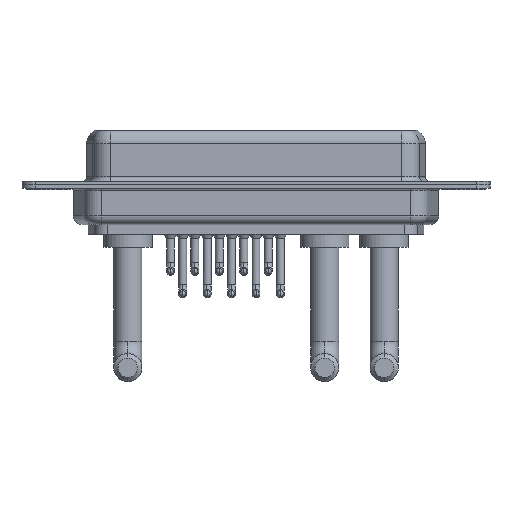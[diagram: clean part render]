
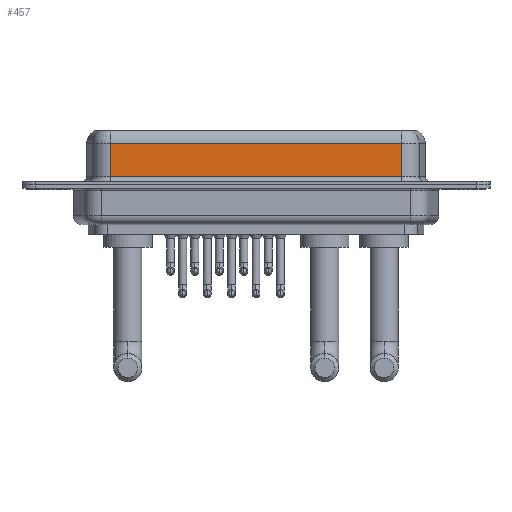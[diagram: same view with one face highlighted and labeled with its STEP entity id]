
A CAD part, front view. The second image highlights one B-rep face of the part: STEP entity #457.
In plain terms, the highlighted planar face has unit normal (0, -1, 0).
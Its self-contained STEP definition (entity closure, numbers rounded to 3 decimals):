
#300 = DIRECTION ( 'NONE',  ( 0., 0., -1. ) ) ;
#441 = DIRECTION ( 'NONE',  ( 0., 0., 1. ) ) ;
#457 = ADVANCED_FACE ( 'NONE', ( #12414 ), #14989, .F. ) ;
#1763 = VERTEX_POINT ( 'NONE', #4613 ) ;
#1808 = EDGE_CURVE ( 'NONE', #10201, #1763, #4521, .T. ) ;
#1873 = VERTEX_POINT ( 'NONE', #11713 ) ;
#2832 = CARTESIAN_POINT ( 'NONE',  ( 40.037, -3.95, 0.9 ) ) ;
#3030 = CARTESIAN_POINT ( 'NONE',  ( 40.037, -3.95, 4.65 ) ) ;
#3142 = DIRECTION ( 'NONE',  ( -1., 0., 0. ) ) ;
#4521 = LINE ( 'NONE', #9871, #14032 ) ;
#4613 = CARTESIAN_POINT ( 'NONE',  ( 7.013, -3.95, 4.65 ) ) ;
#4950 = ORIENTED_EDGE ( 'NONE', *, *, #7436, .T. ) ;
#4983 = ORIENTED_EDGE ( 'NONE', *, *, #5092, .T. ) ;
#5092 = EDGE_CURVE ( 'NONE', #1873, #16533, #16249, .T. ) ;
#6666 = DIRECTION ( 'NONE',  ( 0., 0., -1. ) ) ;
#6929 = LINE ( 'NONE', #10951, #16911 ) ;
#7233 = DIRECTION ( 'NONE',  ( 0., 1., 0. ) ) ;
#7436 = EDGE_CURVE ( 'NONE', #1763, #1873, #13238, .T. ) ;
#9547 = DIRECTION ( 'NONE',  ( 1., 0., 0. ) ) ;
#9871 = CARTESIAN_POINT ( 'NONE',  ( 40.037, -3.95, 4.65 ) ) ;
#10201 = VERTEX_POINT ( 'NONE', #3030 ) ;
#10709 = EDGE_CURVE ( 'NONE', #10201, #16533, #6929, .T. ) ;
#10951 = CARTESIAN_POINT ( 'NONE',  ( 40.037, -3.95, 6.4 ) ) ;
#11713 = CARTESIAN_POINT ( 'NONE',  ( 7.013, -3.95, 0.9 ) ) ;
#11743 = ORIENTED_EDGE ( 'NONE', *, *, #10709, .F. ) ;
#11939 = EDGE_LOOP ( 'NONE', ( #11743, #14622, #4950, #4983 ) ) ;
#12414 = FACE_OUTER_BOUND ( 'NONE', #11939, .T. ) ;
#13208 = AXIS2_PLACEMENT_3D ( 'NONE', #13943, #7233, #441 ) ;
#13238 = LINE ( 'NONE', #14613, #15450 ) ;
#13943 = CARTESIAN_POINT ( 'NONE',  ( 40.037, -3.95, 6.4 ) ) ;
#14032 = VECTOR ( 'NONE', #3142, 1000. ) ;
#14613 = CARTESIAN_POINT ( 'NONE',  ( 7.013, -3.95, 6.4 ) ) ;
#14622 = ORIENTED_EDGE ( 'NONE', *, *, #1808, .T. ) ;
#14989 = PLANE ( 'NONE',  #13208 ) ;
#15450 = VECTOR ( 'NONE', #6666, 1000. ) ;
#15629 = CARTESIAN_POINT ( 'NONE',  ( 40.037, -3.95, 0.9 ) ) ;
#16249 = LINE ( 'NONE', #2832, #16752 ) ;
#16533 = VERTEX_POINT ( 'NONE', #15629 ) ;
#16752 = VECTOR ( 'NONE', #9547, 1000. ) ;
#16911 = VECTOR ( 'NONE', #300, 1000. ) ;
